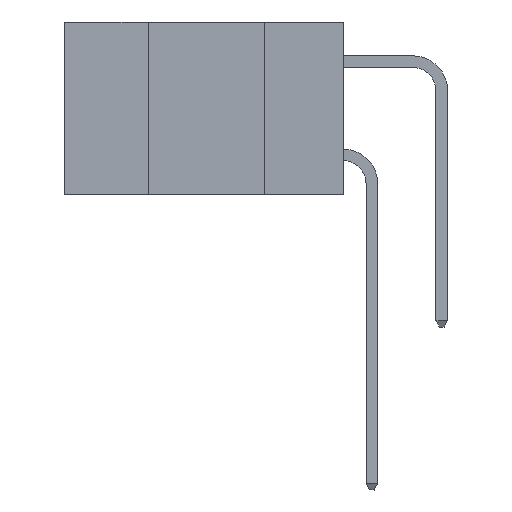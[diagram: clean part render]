
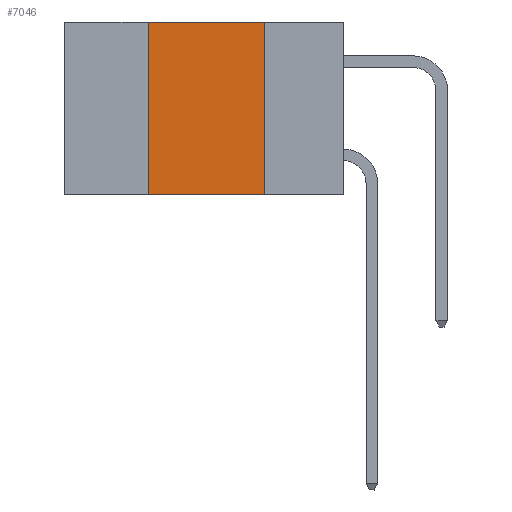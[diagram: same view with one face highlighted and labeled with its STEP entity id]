
A CAD part, left-side view. The second image highlights one B-rep face of the part: STEP entity #7046.
In plain terms, the highlighted planar face has unit normal (-1, 0, 0).
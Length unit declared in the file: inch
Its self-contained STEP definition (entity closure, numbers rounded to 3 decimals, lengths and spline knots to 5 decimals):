
#365 = CARTESIAN_POINT ( 'NONE',  ( 0., 0.6, -0.37 ) ) ;
#918 = ORIENTED_EDGE ( 'NONE', *, *, #3474, .F. ) ;
#3474 = EDGE_CURVE ( 'NONE', #27527, #5140, #18747, .T. ) ;
#4131 = VERTEX_POINT ( 'NONE', #9119 ) ;
#4699 = PLANE ( 'NONE',  #8954 ) ;
#5124 = VECTOR ( 'NONE', #13931, 39.37008 ) ;
#5136 = CARTESIAN_POINT ( 'NONE',  ( 0., 0.17, -0.37 ) ) ;
#5140 = VERTEX_POINT ( 'NONE', #16471 ) ;
#5883 = DIRECTION ( 'NONE',  ( 0., -1., 0. ) ) ;
#6773 = ORIENTED_EDGE ( 'NONE', *, *, #27452, .F. ) ;
#6889 = DIRECTION ( 'NONE',  ( 0., -1., 0. ) ) ;
#7046 = ADVANCED_FACE ( 'NONE', ( #13070 ), #4699, .F. ) ;
#8954 = AXIS2_PLACEMENT_3D ( 'NONE', #12793, #8967, #21822 ) ;
#8967 = DIRECTION ( 'NONE',  ( 1., 0., 0. ) ) ;
#9119 = CARTESIAN_POINT ( 'NONE',  ( 0., 0.17, -0.37 ) ) ;
#9972 = LINE ( 'NONE', #20975, #18908 ) ;
#12026 = VECTOR ( 'NONE', #5883, 39.37008 ) ;
#12793 = CARTESIAN_POINT ( 'NONE',  ( 0., 0.6, 0. ) ) ;
#12956 = ORIENTED_EDGE ( 'NONE', *, *, #20868, .T. ) ;
#13070 = FACE_OUTER_BOUND ( 'NONE', #18871, .T. ) ;
#13931 = DIRECTION ( 'NONE',  ( 0., 0., -1. ) ) ;
#16471 = CARTESIAN_POINT ( 'NONE',  ( 0., 0.17, 0. ) ) ;
#17739 = ORIENTED_EDGE ( 'NONE', *, *, #19645, .F. ) ;
#18577 = CARTESIAN_POINT ( 'NONE',  ( 0., 0.42, 0. ) ) ;
#18747 = LINE ( 'NONE', #25416, #12026 ) ;
#18871 = EDGE_LOOP ( 'NONE', ( #17739, #918, #6773, #12956 ) ) ;
#18908 = VECTOR ( 'NONE', #20427, 39.37008 ) ;
#19645 = EDGE_CURVE ( 'NONE', #5140, #4131, #20560, .T. ) ;
#19740 = LINE ( 'NONE', #365, #24140 ) ;
#20278 = VERTEX_POINT ( 'NONE', #27871 ) ;
#20427 = DIRECTION ( 'NONE',  ( 0., 0., 1. ) ) ;
#20560 = LINE ( 'NONE', #5136, #5124 ) ;
#20868 = EDGE_CURVE ( 'NONE', #20278, #4131, #19740, .T. ) ;
#20975 = CARTESIAN_POINT ( 'NONE',  ( 0., 0.42, -0.37 ) ) ;
#21822 = DIRECTION ( 'NONE',  ( 0., 0., -1. ) ) ;
#24140 = VECTOR ( 'NONE', #6889, 39.37008 ) ;
#25416 = CARTESIAN_POINT ( 'NONE',  ( 0., 0.6, 0. ) ) ;
#27452 = EDGE_CURVE ( 'NONE', #20278, #27527, #9972, .T. ) ;
#27527 = VERTEX_POINT ( 'NONE', #18577 ) ;
#27871 = CARTESIAN_POINT ( 'NONE',  ( 0., 0.42, -0.37 ) ) ;
